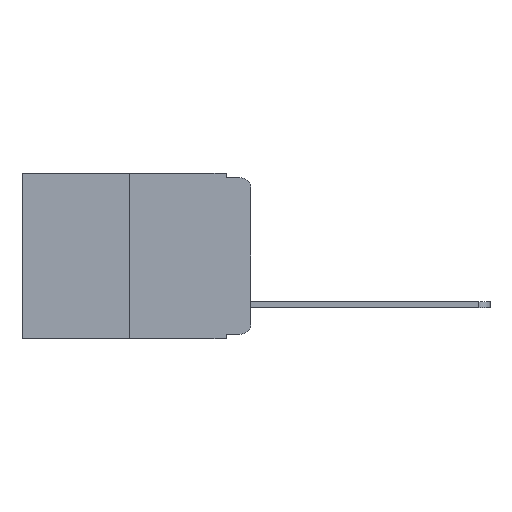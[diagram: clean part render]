
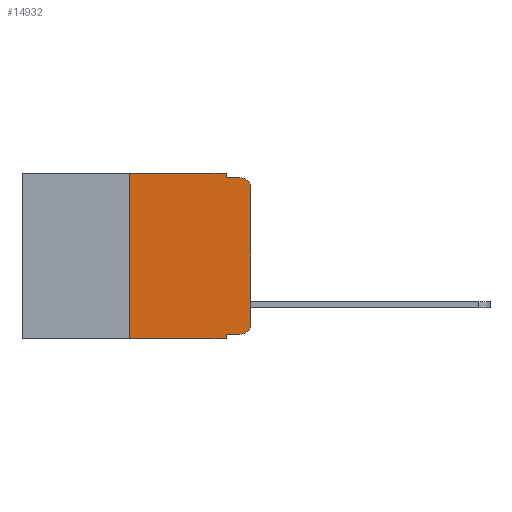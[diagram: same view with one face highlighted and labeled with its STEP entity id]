
A CAD part, left-side view. The second image highlights one B-rep face of the part: STEP entity #14932.
In plain terms, the highlighted planar face has unit normal (-1, 0, 0).
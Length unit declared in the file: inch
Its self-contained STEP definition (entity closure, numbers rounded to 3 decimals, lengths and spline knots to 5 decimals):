
#203 = DIRECTION ( 'NONE',  ( 0., -1., 0. ) ) ;
#259 = VECTOR ( 'NONE', #16968, 39.37008 ) ;
#305 = CARTESIAN_POINT ( 'NONE',  ( 0., 0.02, -0.01 ) ) ;
#360 = DIRECTION ( 'NONE',  ( 0., -1., 0. ) ) ;
#532 = ORIENTED_EDGE ( 'NONE', *, *, #11712, .T. ) ;
#863 = EDGE_CURVE ( 'NONE', #17378, #18425, #18002, .T. ) ;
#875 = ORIENTED_EDGE ( 'NONE', *, *, #11192, .T. ) ;
#1068 = PLANE ( 'NONE',  #4757 ) ;
#1085 = ORIENTED_EDGE ( 'NONE', *, *, #863, .T. ) ;
#1454 = LINE ( 'NONE', #7846, #8155 ) ;
#1494 = EDGE_CURVE ( 'NONE', #1913, #2844, #1454, .T. ) ;
#1663 = FACE_OUTER_BOUND ( 'NONE', #16175, .T. ) ;
#1913 = VERTEX_POINT ( 'NONE', #6018 ) ;
#1941 = VERTEX_POINT ( 'NONE', #11187 ) ;
#2067 = CARTESIAN_POINT ( 'NONE',  ( 0., 0.02, -0.333 ) ) ;
#2360 = CARTESIAN_POINT ( 'NONE',  ( 0., 0.25, -0.343 ) ) ;
#2844 = VERTEX_POINT ( 'NONE', #21093 ) ;
#3285 = VECTOR ( 'NONE', #7803, 39.37008 ) ;
#3500 = LINE ( 'NONE', #8361, #259 ) ;
#3535 = CARTESIAN_POINT ( 'NONE',  ( 0., 0.02, -0.03 ) ) ;
#3981 = VERTEX_POINT ( 'NONE', #305 ) ;
#4012 = CARTESIAN_POINT ( 'NONE',  ( 0., 0.051, 0. ) ) ;
#4517 = DIRECTION ( 'NONE',  ( 0., 0., -1. ) ) ;
#4562 = LINE ( 'NONE', #7108, #12266 ) ;
#4757 = AXIS2_PLACEMENT_3D ( 'NONE', #6158, #14689, #4517 ) ;
#4791 = EDGE_CURVE ( 'NONE', #17378, #17818, #8843, .T. ) ;
#4891 = CARTESIAN_POINT ( 'NONE',  ( 0., 0.02, -0.313 ) ) ;
#5265 = VECTOR ( 'NONE', #9125, 39.37008 ) ;
#5710 = AXIS2_PLACEMENT_3D ( 'NONE', #4891, #9920, #6543 ) ;
#5744 = EDGE_CURVE ( 'NONE', #19345, #3981, #4562, .T. ) ;
#6018 = CARTESIAN_POINT ( 'NONE',  ( 0., 0., -0.313 ) ) ;
#6158 = CARTESIAN_POINT ( 'NONE',  ( 0., 0.473, 0. ) ) ;
#6413 = DIRECTION ( 'NONE',  ( 0., 0., 1. ) ) ;
#6543 = DIRECTION ( 'NONE',  ( 0., 0., -1. ) ) ;
#6724 = AXIS2_PLACEMENT_3D ( 'NONE', #3535, #10277, #13704 ) ;
#7108 = CARTESIAN_POINT ( 'NONE',  ( 0., 0.051, -0.01 ) ) ;
#7751 = CARTESIAN_POINT ( 'NONE',  ( 0., 0.25, 0. ) ) ;
#7803 = DIRECTION ( 'NONE',  ( 0., -1., 0. ) ) ;
#7846 = CARTESIAN_POINT ( 'NONE',  ( 0., 0., 0. ) ) ;
#8155 = VECTOR ( 'NONE', #6413, 39.37008 ) ;
#8191 = LINE ( 'NONE', #17951, #13996 ) ;
#8361 = CARTESIAN_POINT ( 'NONE',  ( 0., 0.051, 0. ) ) ;
#8462 = CIRCLE ( 'NONE', #5710, 0.02 ) ;
#8843 = LINE ( 'NONE', #4012, #10138 ) ;
#8884 = CARTESIAN_POINT ( 'NONE',  ( 0., 0.051, -0.333 ) ) ;
#9125 = DIRECTION ( 'NONE',  ( 0., 0., 1. ) ) ;
#9584 = EDGE_CURVE ( 'NONE', #10989, #13935, #16182, .T. ) ;
#9920 = DIRECTION ( 'NONE',  ( -1., 0., 0. ) ) ;
#10138 = VECTOR ( 'NONE', #19302, 39.37008 ) ;
#10277 = DIRECTION ( 'NONE',  ( -1., 0., 0. ) ) ;
#10595 = ORIENTED_EDGE ( 'NONE', *, *, #1494, .T. ) ;
#10989 = VERTEX_POINT ( 'NONE', #2360 ) ;
#11187 = CARTESIAN_POINT ( 'NONE',  ( 0., 0.051, 0. ) ) ;
#11192 = EDGE_CURVE ( 'NONE', #18425, #1913, #8462, .T. ) ;
#11464 = DIRECTION ( 'NONE',  ( 0., -1., 0. ) ) ;
#11712 = EDGE_CURVE ( 'NONE', #10989, #17818, #8191, .T. ) ;
#12266 = VECTOR ( 'NONE', #203, 39.37008 ) ;
#12811 = CARTESIAN_POINT ( 'NONE',  ( 0., 0.051, -0.333 ) ) ;
#13448 = VECTOR ( 'NONE', #360, 39.37008 ) ;
#13520 = EDGE_CURVE ( 'NONE', #2844, #3981, #15283, .T. ) ;
#13704 = DIRECTION ( 'NONE',  ( 0., 0., -1. ) ) ;
#13935 = VERTEX_POINT ( 'NONE', #21423 ) ;
#13996 = VECTOR ( 'NONE', #11464, 39.37008 ) ;
#14689 = DIRECTION ( 'NONE',  ( 1., 0., 0. ) ) ;
#14854 = EDGE_CURVE ( 'NONE', #13935, #1941, #17631, .T. ) ;
#14932 = ADVANCED_FACE ( 'NONE', ( #1663 ), #1068, .F. ) ;
#15099 = ORIENTED_EDGE ( 'NONE', *, *, #9584, .F. ) ;
#15283 = CIRCLE ( 'NONE', #6724, 0.02 ) ;
#15914 = EDGE_CURVE ( 'NONE', #1941, #19345, #3500, .T. ) ;
#15917 = CARTESIAN_POINT ( 'NONE',  ( 0., 0.051, -0.343 ) ) ;
#16175 = EDGE_LOOP ( 'NONE', ( #10595, #16284, #18874, #20028, #19245, #15099, #532, #17450, #1085, #875 ) ) ;
#16182 = LINE ( 'NONE', #7751, #5265 ) ;
#16284 = ORIENTED_EDGE ( 'NONE', *, *, #13520, .T. ) ;
#16968 = DIRECTION ( 'NONE',  ( 0., 0., -1. ) ) ;
#17378 = VERTEX_POINT ( 'NONE', #8884 ) ;
#17450 = ORIENTED_EDGE ( 'NONE', *, *, #4791, .F. ) ;
#17631 = LINE ( 'NONE', #17880, #3285 ) ;
#17649 = CARTESIAN_POINT ( 'NONE',  ( 0., 0.051, -0.01 ) ) ;
#17818 = VERTEX_POINT ( 'NONE', #15917 ) ;
#17880 = CARTESIAN_POINT ( 'NONE',  ( 0., 0.473, 0. ) ) ;
#17951 = CARTESIAN_POINT ( 'NONE',  ( 0., 0.473, -0.343 ) ) ;
#18002 = LINE ( 'NONE', #12811, #13448 ) ;
#18425 = VERTEX_POINT ( 'NONE', #2067 ) ;
#18874 = ORIENTED_EDGE ( 'NONE', *, *, #5744, .F. ) ;
#19245 = ORIENTED_EDGE ( 'NONE', *, *, #14854, .F. ) ;
#19302 = DIRECTION ( 'NONE',  ( 0., 0., -1. ) ) ;
#19345 = VERTEX_POINT ( 'NONE', #17649 ) ;
#20028 = ORIENTED_EDGE ( 'NONE', *, *, #15914, .F. ) ;
#21093 = CARTESIAN_POINT ( 'NONE',  ( 0., 0., -0.03 ) ) ;
#21423 = CARTESIAN_POINT ( 'NONE',  ( 0., 0.25, 0. ) ) ;
